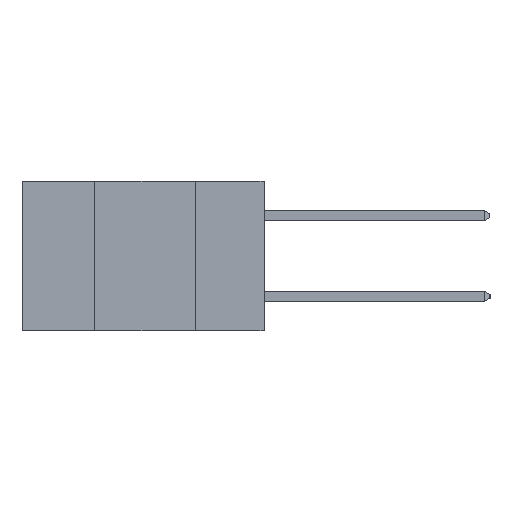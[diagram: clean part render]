
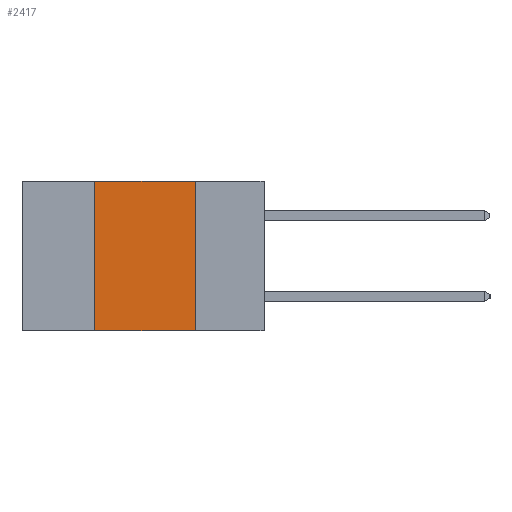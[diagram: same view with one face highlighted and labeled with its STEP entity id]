
A CAD part, left-side view. The second image highlights one B-rep face of the part: STEP entity #2417.
In plain terms, the highlighted planar face has unit normal (-1, 0, 0).
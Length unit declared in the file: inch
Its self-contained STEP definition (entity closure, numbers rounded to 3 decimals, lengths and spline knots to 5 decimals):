
#160 = CARTESIAN_POINT ( 'NONE',  ( 0., 0.6, 0. ) ) ;
#549 = VERTEX_POINT ( 'NONE', #14929 ) ;
#1075 = ORIENTED_EDGE ( 'NONE', *, *, #1311, .F. ) ;
#1311 = EDGE_CURVE ( 'NONE', #10706, #549, #25772, .T. ) ;
#2417 = ADVANCED_FACE ( 'NONE', ( #16752 ), #24190, .F. ) ;
#2960 = VECTOR ( 'NONE', #9568, 39.37008 ) ;
#3326 = CARTESIAN_POINT ( 'NONE',  ( 0., 0.42, -0.37 ) ) ;
#4956 = VERTEX_POINT ( 'NONE', #5007 ) ;
#5007 = CARTESIAN_POINT ( 'NONE',  ( 0., 0.42, -0.37 ) ) ;
#6826 = ORIENTED_EDGE ( 'NONE', *, *, #7500, .F. ) ;
#7135 = EDGE_CURVE ( 'NONE', #4956, #26138, #26798, .T. ) ;
#7500 = EDGE_CURVE ( 'NONE', #26138, #10706, #13019, .T. ) ;
#9568 = DIRECTION ( 'NONE',  ( 0., -1., 0. ) ) ;
#9829 = DIRECTION ( 'NONE',  ( 0., 0., -1. ) ) ;
#10706 = VERTEX_POINT ( 'NONE', #15052 ) ;
#11102 = CARTESIAN_POINT ( 'NONE',  ( 0., 0.17, -0.37 ) ) ;
#11792 = DIRECTION ( 'NONE',  ( 0., 0., 1. ) ) ;
#12772 = DIRECTION ( 'NONE',  ( 0., -1., 0. ) ) ;
#13019 = LINE ( 'NONE', #160, #17822 ) ;
#14929 = CARTESIAN_POINT ( 'NONE',  ( 0., 0.17, -0.37 ) ) ;
#15052 = CARTESIAN_POINT ( 'NONE',  ( 0., 0.17, 0. ) ) ;
#16331 = CARTESIAN_POINT ( 'NONE',  ( 0., 0.42, 0. ) ) ;
#16752 = FACE_OUTER_BOUND ( 'NONE', #20528, .T. ) ;
#17028 = EDGE_CURVE ( 'NONE', #4956, #549, #24976, .T. ) ;
#17822 = VECTOR ( 'NONE', #12772, 39.37008 ) ;
#19577 = ORIENTED_EDGE ( 'NONE', *, *, #17028, .T. ) ;
#20357 = VECTOR ( 'NONE', #9829, 39.37008 ) ;
#20528 = EDGE_LOOP ( 'NONE', ( #1075, #6826, #24098, #19577 ) ) ;
#21375 = VECTOR ( 'NONE', #11792, 39.37008 ) ;
#23960 = CARTESIAN_POINT ( 'NONE',  ( 0., 0.6, -0.37 ) ) ;
#23961 = DIRECTION ( 'NONE',  ( 0., 0., -1. ) ) ;
#23999 = DIRECTION ( 'NONE',  ( 1., 0., 0. ) ) ;
#24098 = ORIENTED_EDGE ( 'NONE', *, *, #7135, .F. ) ;
#24103 = CARTESIAN_POINT ( 'NONE',  ( 0., 0.6, 0. ) ) ;
#24190 = PLANE ( 'NONE',  #25745 ) ;
#24976 = LINE ( 'NONE', #23960, #2960 ) ;
#25745 = AXIS2_PLACEMENT_3D ( 'NONE', #24103, #23999, #23961 ) ;
#25772 = LINE ( 'NONE', #11102, #20357 ) ;
#26138 = VERTEX_POINT ( 'NONE', #16331 ) ;
#26798 = LINE ( 'NONE', #3326, #21375 ) ;
